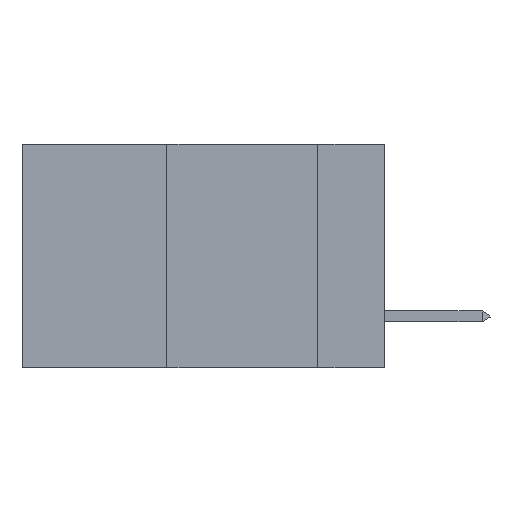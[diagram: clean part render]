
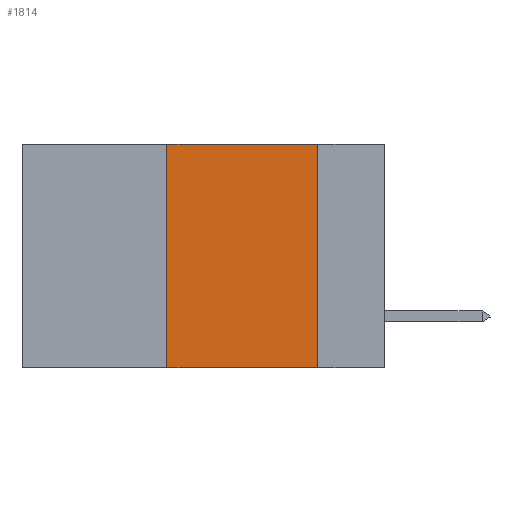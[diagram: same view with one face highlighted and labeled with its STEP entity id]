
A CAD part, left-side view. The second image highlights one B-rep face of the part: STEP entity #1814.
In plain terms, the highlighted planar face has unit normal (-1, 0, 0).
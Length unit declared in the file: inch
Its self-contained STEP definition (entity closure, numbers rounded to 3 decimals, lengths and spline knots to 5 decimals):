
#1097 = CARTESIAN_POINT ( 'NONE',  ( 0., 0.11, -0.37 ) ) ;
#1584 = VERTEX_POINT ( 'NONE', #9235 ) ;
#1814 = ADVANCED_FACE ( 'NONE', ( #20027 ), #29364, .F. ) ;
#4205 = ORIENTED_EDGE ( 'NONE', *, *, #22280, .T. ) ;
#6055 = DIRECTION ( 'NONE',  ( 0., 0., -1. ) ) ;
#6275 = CARTESIAN_POINT ( 'NONE',  ( 0., 0.11, 0. ) ) ;
#9009 = ORIENTED_EDGE ( 'NONE', *, *, #30209, .F. ) ;
#9162 = VERTEX_POINT ( 'NONE', #6275 ) ;
#9235 = CARTESIAN_POINT ( 'NONE',  ( 0., 0.36, -0.37 ) ) ;
#10136 = CARTESIAN_POINT ( 'NONE',  ( 0., 0.6, 0. ) ) ;
#11855 = CARTESIAN_POINT ( 'NONE',  ( 0., 0.36, 0. ) ) ;
#12682 = AXIS2_PLACEMENT_3D ( 'NONE', #10136, #24841, #14644 ) ;
#13493 = VERTEX_POINT ( 'NONE', #1097 ) ;
#14644 = DIRECTION ( 'NONE',  ( 0., 0., -1. ) ) ;
#15654 = CARTESIAN_POINT ( 'NONE',  ( 0., 0.6, -0.37 ) ) ;
#16198 = ORIENTED_EDGE ( 'NONE', *, *, #18938, .F. ) ;
#16237 = LINE ( 'NONE', #11855, #30077 ) ;
#16288 = CARTESIAN_POINT ( 'NONE',  ( 0., 0.36, 0. ) ) ;
#16332 = VERTEX_POINT ( 'NONE', #16288 ) ;
#16395 = LINE ( 'NONE', #15654, #25606 ) ;
#16723 = CARTESIAN_POINT ( 'NONE',  ( 0., 0.6, 0. ) ) ;
#18938 = EDGE_CURVE ( 'NONE', #1584, #16332, #16237, .T. ) ;
#19524 = EDGE_LOOP ( 'NONE', ( #9009, #29404, #16198, #4205 ) ) ;
#20027 = FACE_OUTER_BOUND ( 'NONE', #19524, .T. ) ;
#21761 = LINE ( 'NONE', #25290, #29423 ) ;
#22280 = EDGE_CURVE ( 'NONE', #1584, #13493, #16395, .T. ) ;
#24841 = DIRECTION ( 'NONE',  ( 1., 0., 0. ) ) ;
#25077 = LINE ( 'NONE', #16723, #27793 ) ;
#25290 = CARTESIAN_POINT ( 'NONE',  ( 0., 0.11, 0. ) ) ;
#25606 = VECTOR ( 'NONE', #27606, 39.37008 ) ;
#27606 = DIRECTION ( 'NONE',  ( 0., -1., 0. ) ) ;
#27793 = VECTOR ( 'NONE', #31619, 39.37008 ) ;
#29231 = DIRECTION ( 'NONE',  ( 0., 0., 1. ) ) ;
#29364 = PLANE ( 'NONE',  #12682 ) ;
#29404 = ORIENTED_EDGE ( 'NONE', *, *, #31641, .F. ) ;
#29423 = VECTOR ( 'NONE', #6055, 39.37008 ) ;
#30077 = VECTOR ( 'NONE', #29231, 39.37008 ) ;
#30209 = EDGE_CURVE ( 'NONE', #9162, #13493, #21761, .T. ) ;
#31619 = DIRECTION ( 'NONE',  ( 0., -1., 0. ) ) ;
#31641 = EDGE_CURVE ( 'NONE', #16332, #9162, #25077, .T. ) ;
